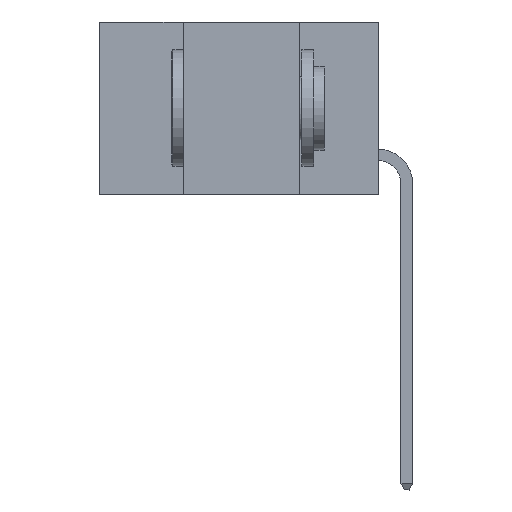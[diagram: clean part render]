
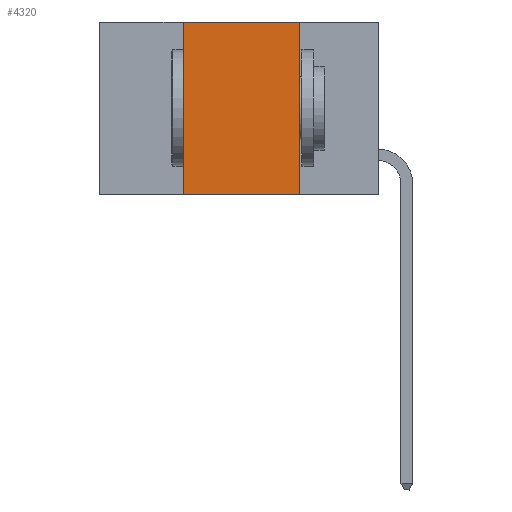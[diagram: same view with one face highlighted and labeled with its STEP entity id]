
A CAD part, left-side view. The second image highlights one B-rep face of the part: STEP entity #4320.
In plain terms, the highlighted planar face has unit normal (-1, 0, 0).
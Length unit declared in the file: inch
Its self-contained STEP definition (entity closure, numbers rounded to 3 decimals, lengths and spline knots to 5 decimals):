
#117 = EDGE_CURVE ( 'NONE', #3859, #3178, #9143, .T. ) ;
#134 = PLANE ( 'NONE',  #1901 ) ;
#240 = VECTOR ( 'NONE', #5629, 39.37008 ) ;
#568 = CARTESIAN_POINT ( 'NONE',  ( 0., 0.42, -0.37 ) ) ;
#816 = LINE ( 'NONE', #2787, #3849 ) ;
#887 = ORIENTED_EDGE ( 'NONE', *, *, #5632, .F. ) ;
#1028 = LINE ( 'NONE', #8758, #2936 ) ;
#1473 = CARTESIAN_POINT ( 'NONE',  ( 0., 0.6, 0. ) ) ;
#1901 = AXIS2_PLACEMENT_3D ( 'NONE', #3750, #6431, #7132 ) ;
#2185 = CARTESIAN_POINT ( 'NONE',  ( 0., 0.17, 0. ) ) ;
#2675 = DIRECTION ( 'NONE',  ( 0., 0., 1. ) ) ;
#2711 = LINE ( 'NONE', #568, #8857 ) ;
#2787 = CARTESIAN_POINT ( 'NONE',  ( 0., 0.6, -0.37 ) ) ;
#2936 = VECTOR ( 'NONE', #5383, 39.37008 ) ;
#3178 = VERTEX_POINT ( 'NONE', #2185 ) ;
#3491 = DIRECTION ( 'NONE',  ( 0., -1., 0. ) ) ;
#3750 = CARTESIAN_POINT ( 'NONE',  ( 0., 0.6, 0. ) ) ;
#3849 = VECTOR ( 'NONE', #3491, 39.37008 ) ;
#3859 = VERTEX_POINT ( 'NONE', #7797 ) ;
#4320 = ADVANCED_FACE ( 'NONE', ( #8702 ), #134, .F. ) ;
#5383 = DIRECTION ( 'NONE',  ( 0., 0., -1. ) ) ;
#5629 = DIRECTION ( 'NONE',  ( 0., -1., 0. ) ) ;
#5632 = EDGE_CURVE ( 'NONE', #8152, #3859, #2711, .T. ) ;
#6050 = EDGE_LOOP ( 'NONE', ( #6491, #7963, #887, #6642 ) ) ;
#6100 = CARTESIAN_POINT ( 'NONE',  ( 0., 0.17, -0.37 ) ) ;
#6431 = DIRECTION ( 'NONE',  ( 1., 0., 0. ) ) ;
#6491 = ORIENTED_EDGE ( 'NONE', *, *, #8045, .F. ) ;
#6642 = ORIENTED_EDGE ( 'NONE', *, *, #8765, .T. ) ;
#7132 = DIRECTION ( 'NONE',  ( 0., 0., -1. ) ) ;
#7733 = CARTESIAN_POINT ( 'NONE',  ( 0., 0.42, -0.37 ) ) ;
#7797 = CARTESIAN_POINT ( 'NONE',  ( 0., 0.42, 0. ) ) ;
#7963 = ORIENTED_EDGE ( 'NONE', *, *, #117, .F. ) ;
#8045 = EDGE_CURVE ( 'NONE', #3178, #8571, #1028, .T. ) ;
#8152 = VERTEX_POINT ( 'NONE', #7733 ) ;
#8571 = VERTEX_POINT ( 'NONE', #6100 ) ;
#8702 = FACE_OUTER_BOUND ( 'NONE', #6050, .T. ) ;
#8758 = CARTESIAN_POINT ( 'NONE',  ( 0., 0.17, -0.37 ) ) ;
#8765 = EDGE_CURVE ( 'NONE', #8152, #8571, #816, .T. ) ;
#8857 = VECTOR ( 'NONE', #2675, 39.37008 ) ;
#9143 = LINE ( 'NONE', #1473, #240 ) ;
